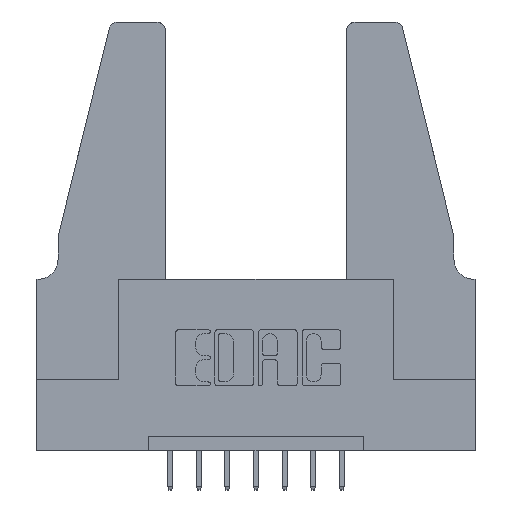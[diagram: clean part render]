
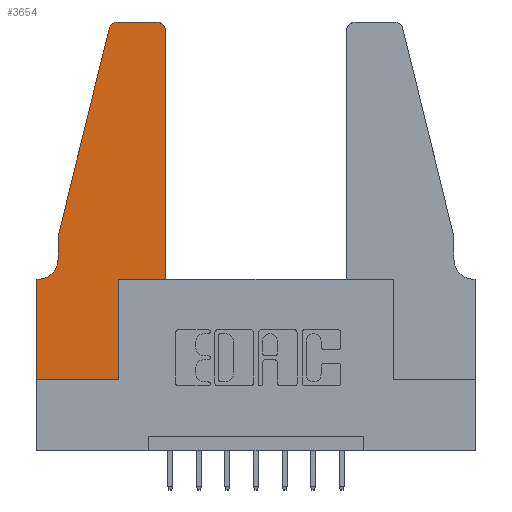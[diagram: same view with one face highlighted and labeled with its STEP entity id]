
A CAD part, top view. The second image highlights one B-rep face of the part: STEP entity #3654.
In plain terms, the highlighted planar face has unit normal (0, 0, 1).
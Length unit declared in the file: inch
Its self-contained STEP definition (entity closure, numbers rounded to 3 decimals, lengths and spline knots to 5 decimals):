
#279 = CARTESIAN_POINT ( 'NONE',  ( 0.0055, 0.35, 0.37 ) ) ;
#316 = ORIENTED_EDGE ( 'NONE', *, *, #5980, .T. ) ;
#319 = DIRECTION ( 'NONE',  ( -1., 0., 0. ) ) ;
#419 = ORIENTED_EDGE ( 'NONE', *, *, #922, .T. ) ;
#723 = CARTESIAN_POINT ( 'NONE',  ( 0., 0.35, 0.37 ) ) ;
#766 = CARTESIAN_POINT ( 'NONE',  ( 0.25487, 1.22718, 0.37 ) ) ;
#882 = DIRECTION ( 'NONE',  ( 1., 0., 0. ) ) ;
#922 = EDGE_CURVE ( 'NONE', #11055, #7515, #7573, .T. ) ;
#966 = CARTESIAN_POINT ( 'NONE',  ( 0.4505, 0.35, 0.37 ) ) ;
#995 = ORIENTED_EDGE ( 'NONE', *, *, #5286, .T. ) ;
#1052 = VERTEX_POINT ( 'NONE', #6762 ) ;
#1084 = EDGE_CURVE ( 'NONE', #8689, #3186, #6703, .T. ) ;
#1224 = CARTESIAN_POINT ( 'NONE',  ( 0.0055, 0.42, 0.37 ) ) ;
#1307 = VECTOR ( 'NONE', #11336, 39.37008 ) ;
#1495 = AXIS2_PLACEMENT_3D ( 'NONE', #9838, #10947, #7084 ) ;
#1716 = EDGE_CURVE ( 'NONE', #10249, #1052, #4638, .T. ) ;
#1724 = DIRECTION ( 'NONE',  ( 1., 0., 0. ) ) ;
#1774 = PLANE ( 'NONE',  #5631 ) ;
#1925 = EDGE_CURVE ( 'NONE', #7515, #7604, #10785, .T. ) ;
#2001 = CARTESIAN_POINT ( 'NONE',  ( 0., 0., 0.37 ) ) ;
#2298 = AXIS2_PLACEMENT_3D ( 'NONE', #1224, #11464, #319 ) ;
#2510 = LINE ( 'NONE', #12047, #5772 ) ;
#2589 = CARTESIAN_POINT ( 'NONE',  ( 0.0755, 0.35, 0.37 ) ) ;
#2641 = VECTOR ( 'NONE', #10509, 39.37008 ) ;
#2721 = LINE ( 'NONE', #7426, #6555 ) ;
#2889 = VECTOR ( 'NONE', #3776, 39.37008 ) ;
#3150 = ORIENTED_EDGE ( 'NONE', *, *, #4933, .T. ) ;
#3186 = VERTEX_POINT ( 'NONE', #10280 ) ;
#3291 = AXIS2_PLACEMENT_3D ( 'NONE', #12071, #8326, #6340 ) ;
#3463 = EDGE_CURVE ( 'NONE', #7604, #8689, #6413, .T. ) ;
#3638 = CARTESIAN_POINT ( 'NONE',  ( 0.4205, 1.25, 0.37 ) ) ;
#3654 = ADVANCED_FACE ( 'NONE', ( #10386 ), #1774, .T. ) ;
#3776 = DIRECTION ( 'NONE',  ( 0., -1., 0. ) ) ;
#4118 = VERTEX_POINT ( 'NONE', #10441 ) ;
#4132 = VERTEX_POINT ( 'NONE', #279 ) ;
#4638 = LINE ( 'NONE', #11053, #4773 ) ;
#4717 = DIRECTION ( 'NONE',  ( 0., -1., 0. ) ) ;
#4764 = VECTOR ( 'NONE', #4717, 39.37008 ) ;
#4773 = VECTOR ( 'NONE', #882, 39.37008 ) ;
#4933 = EDGE_CURVE ( 'NONE', #4118, #10526, #12168, .T. ) ;
#5247 = CARTESIAN_POINT ( 'NONE',  ( 0.4505, 0.35, 0.37 ) ) ;
#5286 = EDGE_CURVE ( 'NONE', #8004, #4118, #2721, .T. ) ;
#5316 = ORIENTED_EDGE ( 'NONE', *, *, #3463, .T. ) ;
#5509 = ORIENTED_EDGE ( 'NONE', *, *, #1925, .T. ) ;
#5611 = ORIENTED_EDGE ( 'NONE', *, *, #1716, .T. ) ;
#5631 = AXIS2_PLACEMENT_3D ( 'NONE', #5659, #9314, #9445 ) ;
#5659 = CARTESIAN_POINT ( 'NONE',  ( 0., 0.35, 0.37 ) ) ;
#5772 = VECTOR ( 'NONE', #7319, 39.37008 ) ;
#5980 = EDGE_CURVE ( 'NONE', #1052, #11055, #2510, .T. ) ;
#6340 = DIRECTION ( 'NONE',  ( 1., 0., 0. ) ) ;
#6413 = CIRCLE ( 'NONE', #1495, 0.03 ) ;
#6555 = VECTOR ( 'NONE', #12144, 39.37008 ) ;
#6703 = LINE ( 'NONE', #7821, #2641 ) ;
#6762 = CARTESIAN_POINT ( 'NONE',  ( 0.2865, 0., 0.37 ) ) ;
#7084 = DIRECTION ( 'NONE',  ( 1., 0., 0. ) ) ;
#7319 = DIRECTION ( 'NONE',  ( 0., 1., 0. ) ) ;
#7374 = CARTESIAN_POINT ( 'NONE',  ( 0.0755, 0.42, 0.37 ) ) ;
#7426 = CARTESIAN_POINT ( 'NONE',  ( 0.0755, 0.5, 0.37 ) ) ;
#7435 = CIRCLE ( 'NONE', #2298, 0.07 ) ;
#7515 = VERTEX_POINT ( 'NONE', #8002 ) ;
#7532 = LINE ( 'NONE', #2589, #1307 ) ;
#7573 = LINE ( 'NONE', #966, #9530 ) ;
#7604 = VERTEX_POINT ( 'NONE', #8732 ) ;
#7627 = CIRCLE ( 'NONE', #3291, 0.03 ) ;
#7821 = CARTESIAN_POINT ( 'NONE',  ( 0.2605, 1.25, 0.37 ) ) ;
#8002 = CARTESIAN_POINT ( 'NONE',  ( 0.4505, 0.35, 0.37 ) ) ;
#8004 = VERTEX_POINT ( 'NONE', #766 ) ;
#8194 = ORIENTED_EDGE ( 'NONE', *, *, #10706, .T. ) ;
#8260 = ORIENTED_EDGE ( 'NONE', *, *, #1084, .T. ) ;
#8326 = DIRECTION ( 'NONE',  ( 0., 0., 1. ) ) ;
#8638 = ORIENTED_EDGE ( 'NONE', *, *, #11560, .T. ) ;
#8689 = VERTEX_POINT ( 'NONE', #3638 ) ;
#8732 = CARTESIAN_POINT ( 'NONE',  ( 0.4505, 1.22, 0.37 ) ) ;
#8967 = DIRECTION ( 'NONE',  ( 0., 1., 0. ) ) ;
#9077 = CARTESIAN_POINT ( 'NONE',  ( 0.2865, 0.35, 0.37 ) ) ;
#9254 = CARTESIAN_POINT ( 'NONE',  ( 0., 0., 0.37 ) ) ;
#9314 = DIRECTION ( 'NONE',  ( 0., 0., 1. ) ) ;
#9346 = VECTOR ( 'NONE', #8967, 39.37008 ) ;
#9426 = CARTESIAN_POINT ( 'NONE',  ( 0.0755, 0.5, 0.37 ) ) ;
#9445 = DIRECTION ( 'NONE',  ( 1., 0., 0. ) ) ;
#9530 = VECTOR ( 'NONE', #1724, 39.37008 ) ;
#9566 = ORIENTED_EDGE ( 'NONE', *, *, #11150, .T. ) ;
#9838 = CARTESIAN_POINT ( 'NONE',  ( 0.4205, 1.22, 0.37 ) ) ;
#9842 = VERTEX_POINT ( 'NONE', #723 ) ;
#10249 = VERTEX_POINT ( 'NONE', #9254 ) ;
#10280 = CARTESIAN_POINT ( 'NONE',  ( 0.284, 1.25, 0.37 ) ) ;
#10386 = FACE_OUTER_BOUND ( 'NONE', #11511, .T. ) ;
#10441 = CARTESIAN_POINT ( 'NONE',  ( 0.0755, 0.5, 0.37 ) ) ;
#10504 = LINE ( 'NONE', #2001, #4764 ) ;
#10509 = DIRECTION ( 'NONE',  ( -1., 0., 0. ) ) ;
#10526 = VERTEX_POINT ( 'NONE', #7374 ) ;
#10706 = EDGE_CURVE ( 'NONE', #4132, #9842, #7532, .T. ) ;
#10785 = LINE ( 'NONE', #5247, #9346 ) ;
#10886 = EDGE_CURVE ( 'NONE', #10526, #4132, #7435, .T. ) ;
#10947 = DIRECTION ( 'NONE',  ( 0., 0., 1. ) ) ;
#11053 = CARTESIAN_POINT ( 'NONE',  ( 0., 0., 0.37 ) ) ;
#11055 = VERTEX_POINT ( 'NONE', #9077 ) ;
#11150 = EDGE_CURVE ( 'NONE', #3186, #8004, #7627, .T. ) ;
#11336 = DIRECTION ( 'NONE',  ( -1., 0., 0. ) ) ;
#11464 = DIRECTION ( 'NONE',  ( 0., 0., -1. ) ) ;
#11511 = EDGE_LOOP ( 'NONE', ( #8260, #9566, #995, #3150, #11623, #8194, #8638, #5611, #316, #419, #5509, #5316 ) ) ;
#11560 = EDGE_CURVE ( 'NONE', #9842, #10249, #10504, .T. ) ;
#11623 = ORIENTED_EDGE ( 'NONE', *, *, #10886, .T. ) ;
#12047 = CARTESIAN_POINT ( 'NONE',  ( 0.2865, 0.35, 0.37 ) ) ;
#12071 = CARTESIAN_POINT ( 'NONE',  ( 0.284, 1.22, 0.37 ) ) ;
#12144 = DIRECTION ( 'NONE',  ( -0.239, -0.971, 0. ) ) ;
#12168 = LINE ( 'NONE', #9426, #2889 ) ;
